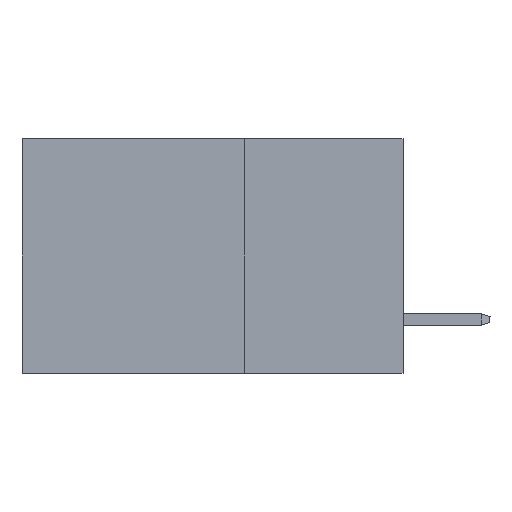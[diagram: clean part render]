
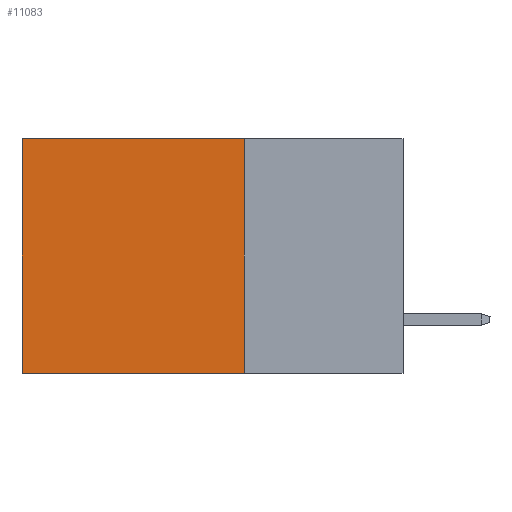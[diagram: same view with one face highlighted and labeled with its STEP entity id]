
A CAD part, left-side view. The second image highlights one B-rep face of the part: STEP entity #11083.
In plain terms, the highlighted planar face has unit normal (-1, 0, 0).
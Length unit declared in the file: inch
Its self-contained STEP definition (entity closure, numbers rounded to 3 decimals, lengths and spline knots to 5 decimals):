
#1726 = VERTEX_POINT ( 'NONE', #38750 ) ;
#2656 = VERTEX_POINT ( 'NONE', #35539 ) ;
#4463 = LINE ( 'NONE', #39840, #7399 ) ;
#4702 = EDGE_LOOP ( 'NONE', ( #14478, #34045, #19395, #34693 ) ) ;
#6596 = VERTEX_POINT ( 'NONE', #18329 ) ;
#7121 = CARTESIAN_POINT ( 'NONE',  ( 0.2875, 0.6, 0. ) ) ;
#7399 = VECTOR ( 'NONE', #21331, 39.37008 ) ;
#8232 = DIRECTION ( 'NONE',  ( 0., 0., -1. ) ) ;
#10316 = VECTOR ( 'NONE', #8232, 39.37008 ) ;
#10785 = FACE_OUTER_BOUND ( 'NONE', #4702, .T. ) ;
#11083 = ADVANCED_FACE ( 'NONE', ( #10785 ), #14045, .F. ) ;
#11694 = CARTESIAN_POINT ( 'NONE',  ( 0.2875, 0.25, 0. ) ) ;
#12866 = AXIS2_PLACEMENT_3D ( 'NONE', #27475, #30940, #40712 ) ;
#13137 = VERTEX_POINT ( 'NONE', #27535 ) ;
#14045 = PLANE ( 'NONE',  #12866 ) ;
#14478 = ORIENTED_EDGE ( 'NONE', *, *, #38989, .T. ) ;
#15050 = DIRECTION ( 'NONE',  ( 0., 1., 0. ) ) ;
#15157 = VECTOR ( 'NONE', #17073, 39.37008 ) ;
#16342 = VECTOR ( 'NONE', #15050, 39.37008 ) ;
#17073 = DIRECTION ( 'NONE',  ( 0., 0., -1. ) ) ;
#18118 = EDGE_CURVE ( 'NONE', #1726, #13137, #34682, .T. ) ;
#18329 = CARTESIAN_POINT ( 'NONE',  ( 0.2875, 0.6, 0. ) ) ;
#19395 = ORIENTED_EDGE ( 'NONE', *, *, #18118, .F. ) ;
#21331 = DIRECTION ( 'NONE',  ( 0., 1., 0. ) ) ;
#23044 = EDGE_CURVE ( 'NONE', #1726, #6596, #39098, .T. ) ;
#27475 = CARTESIAN_POINT ( 'NONE',  ( 0.2875, 0.25, 0. ) ) ;
#27535 = CARTESIAN_POINT ( 'NONE',  ( 0.2875, 0.25, -0.37 ) ) ;
#28904 = CARTESIAN_POINT ( 'NONE',  ( 0.2875, 0.25, 0. ) ) ;
#30940 = DIRECTION ( 'NONE',  ( 1., 0., 0. ) ) ;
#34045 = ORIENTED_EDGE ( 'NONE', *, *, #36633, .F. ) ;
#34682 = LINE ( 'NONE', #11694, #10316 ) ;
#34693 = ORIENTED_EDGE ( 'NONE', *, *, #23044, .T. ) ;
#35539 = CARTESIAN_POINT ( 'NONE',  ( 0.2875, 0.6, -0.37 ) ) ;
#36633 = EDGE_CURVE ( 'NONE', #13137, #2656, #4463, .T. ) ;
#38750 = CARTESIAN_POINT ( 'NONE',  ( 0.2875, 0.25, 0. ) ) ;
#38989 = EDGE_CURVE ( 'NONE', #6596, #2656, #40067, .T. ) ;
#39098 = LINE ( 'NONE', #28904, #16342 ) ;
#39840 = CARTESIAN_POINT ( 'NONE',  ( 0.2875, 0.25, -0.37 ) ) ;
#40067 = LINE ( 'NONE', #7121, #15157 ) ;
#40712 = DIRECTION ( 'NONE',  ( 0., 0., -1. ) ) ;
